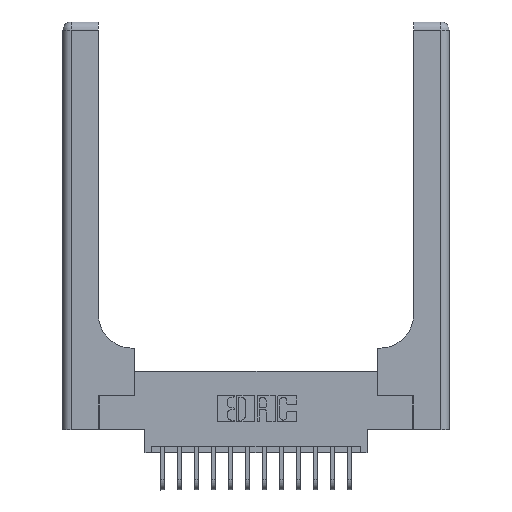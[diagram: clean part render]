
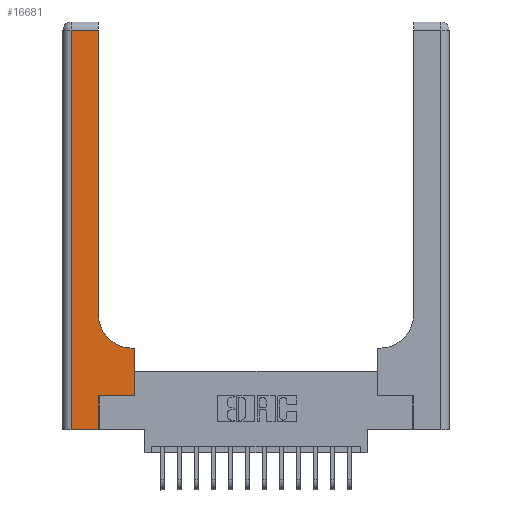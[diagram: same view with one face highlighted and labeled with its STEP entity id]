
A CAD part, top view. The second image highlights one B-rep face of the part: STEP entity #16681.
In plain terms, the highlighted planar face has unit normal (0, 0, 1).
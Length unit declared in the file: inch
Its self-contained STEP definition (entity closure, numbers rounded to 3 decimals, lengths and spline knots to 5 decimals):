
#87 = CARTESIAN_POINT ( 'NONE',  ( 0.528, 0.25, 0.37 ) ) ;
#623 = FACE_OUTER_BOUND ( 'NONE', #810, .T. ) ;
#810 = EDGE_LOOP ( 'NONE', ( #16310, #6818, #9333, #6764, #7889, #3598, #5517, #10188, #7358 ) ) ;
#1104 = LINE ( 'NONE', #11656, #10890 ) ;
#1242 = LINE ( 'NONE', #17725, #15218 ) ;
#1828 = EDGE_CURVE ( 'NONE', #3125, #15995, #2176, .T. ) ;
#2105 = PLANE ( 'NONE',  #14768 ) ;
#2176 = LINE ( 'NONE', #15721, #14375 ) ;
#2318 = DIRECTION ( 'NONE',  ( -1., 0., 0. ) ) ;
#2379 = CARTESIAN_POINT ( 'NONE',  ( 0.06, 2.94, 0.37 ) ) ;
#2805 = CARTESIAN_POINT ( 'NONE',  ( 0.265, 0., 0.37 ) ) ;
#3067 = CARTESIAN_POINT ( 'NONE',  ( 0.265, 0., 0.37 ) ) ;
#3098 = CARTESIAN_POINT ( 'NONE',  ( 0., 0., 0.37 ) ) ;
#3125 = VERTEX_POINT ( 'NONE', #10944 ) ;
#3320 = CARTESIAN_POINT ( 'NONE',  ( 0.26, 2.94, 0.37 ) ) ;
#3598 = ORIENTED_EDGE ( 'NONE', *, *, #18390, .T. ) ;
#4007 = CARTESIAN_POINT ( 'NONE',  ( 0.51, 0.6, 0.37 ) ) ;
#4327 = VERTEX_POINT ( 'NONE', #14497 ) ;
#5517 = ORIENTED_EDGE ( 'NONE', *, *, #10714, .T. ) ;
#5821 = VECTOR ( 'NONE', #13279, 39.37008 ) ;
#6764 = ORIENTED_EDGE ( 'NONE', *, *, #14956, .T. ) ;
#6818 = ORIENTED_EDGE ( 'NONE', *, *, #6959, .T. ) ;
#6959 = EDGE_CURVE ( 'NONE', #15995, #10327, #1104, .T. ) ;
#7268 = VECTOR ( 'NONE', #9680, 39.37008 ) ;
#7292 = DIRECTION ( 'NONE',  ( 0., 0., -1. ) ) ;
#7358 = ORIENTED_EDGE ( 'NONE', *, *, #9539, .T. ) ;
#7841 = VECTOR ( 'NONE', #12265, 39.37008 ) ;
#7850 = EDGE_CURVE ( 'NONE', #10327, #13882, #17471, .T. ) ;
#7889 = ORIENTED_EDGE ( 'NONE', *, *, #10748, .T. ) ;
#8124 = DIRECTION ( 'NONE',  ( 0., 0., -1. ) ) ;
#8308 = CARTESIAN_POINT ( 'NONE',  ( 0.265, 0.25, 0.37 ) ) ;
#8493 = VERTEX_POINT ( 'NONE', #4007 ) ;
#8628 = DIRECTION ( 'NONE',  ( 0., 1., 0. ) ) ;
#8700 = VECTOR ( 'NONE', #2318, 39.37008 ) ;
#9197 = DIRECTION ( 'NONE',  ( -1., 0., 0. ) ) ;
#9333 = ORIENTED_EDGE ( 'NONE', *, *, #7850, .T. ) ;
#9539 = EDGE_CURVE ( 'NONE', #8493, #3125, #19323, .T. ) ;
#9680 = DIRECTION ( 'NONE',  ( 1., 0., 0. ) ) ;
#10188 = ORIENTED_EDGE ( 'NONE', *, *, #11482, .T. ) ;
#10327 = VERTEX_POINT ( 'NONE', #2379 ) ;
#10426 = CARTESIAN_POINT ( 'NONE',  ( 0.06, 0., 0.37 ) ) ;
#10714 = EDGE_CURVE ( 'NONE', #18818, #4327, #1242, .T. ) ;
#10748 = EDGE_CURVE ( 'NONE', #12041, #18580, #17923, .T. ) ;
#10890 = VECTOR ( 'NONE', #16944, 39.37008 ) ;
#10944 = CARTESIAN_POINT ( 'NONE',  ( 0.26, 0.85, 0.37 ) ) ;
#11335 = DIRECTION ( 'NONE',  ( 0., 1., 0. ) ) ;
#11482 = EDGE_CURVE ( 'NONE', #4327, #8493, #15766, .T. ) ;
#11594 = CARTESIAN_POINT ( 'NONE',  ( 0.26, 0.6, 0.37 ) ) ;
#11625 = DIRECTION ( 'NONE',  ( 1., 0., 0. ) ) ;
#11656 = CARTESIAN_POINT ( 'NONE',  ( 0., 2.94, 0.37 ) ) ;
#11733 = CARTESIAN_POINT ( 'NONE',  ( 0.51, 0.85, 0.37 ) ) ;
#12041 = VERTEX_POINT ( 'NONE', #3067 ) ;
#12265 = DIRECTION ( 'NONE',  ( 1., 0., 0. ) ) ;
#12767 = AXIS2_PLACEMENT_3D ( 'NONE', #11733, #7292, #11625 ) ;
#13279 = DIRECTION ( 'NONE',  ( 0., 1., 0. ) ) ;
#13396 = CARTESIAN_POINT ( 'NONE',  ( 0.06, 3., 0.37 ) ) ;
#13712 = CARTESIAN_POINT ( 'NONE',  ( 0.265, 0.25, 0.37 ) ) ;
#13830 = CARTESIAN_POINT ( 'NONE',  ( 0., 3., 0.37 ) ) ;
#13882 = VERTEX_POINT ( 'NONE', #10426 ) ;
#14375 = VECTOR ( 'NONE', #11335, 39.37008 ) ;
#14497 = CARTESIAN_POINT ( 'NONE',  ( 0.528, 0.6, 0.37 ) ) ;
#14644 = DIRECTION ( 'NONE',  ( 0., -1., 0. ) ) ;
#14718 = VECTOR ( 'NONE', #14644, 39.37008 ) ;
#14768 = AXIS2_PLACEMENT_3D ( 'NONE', #13830, #8124, #9197 ) ;
#14956 = EDGE_CURVE ( 'NONE', #13882, #12041, #15449, .T. ) ;
#15218 = VECTOR ( 'NONE', #8628, 39.37008 ) ;
#15449 = LINE ( 'NONE', #3098, #7841 ) ;
#15721 = CARTESIAN_POINT ( 'NONE',  ( 0.26, 3., 0.37 ) ) ;
#15766 = LINE ( 'NONE', #11594, #8700 ) ;
#15995 = VERTEX_POINT ( 'NONE', #3320 ) ;
#16310 = ORIENTED_EDGE ( 'NONE', *, *, #1828, .T. ) ;
#16681 = ADVANCED_FACE ( 'NONE', ( #623 ), #2105, .F. ) ;
#16944 = DIRECTION ( 'NONE',  ( -1., 0., 0. ) ) ;
#17094 = LINE ( 'NONE', #8308, #7268 ) ;
#17471 = LINE ( 'NONE', #13396, #14718 ) ;
#17725 = CARTESIAN_POINT ( 'NONE',  ( 0.528, 0.25, 0.37 ) ) ;
#17923 = LINE ( 'NONE', #2805, #5821 ) ;
#18390 = EDGE_CURVE ( 'NONE', #18580, #18818, #17094, .T. ) ;
#18580 = VERTEX_POINT ( 'NONE', #13712 ) ;
#18818 = VERTEX_POINT ( 'NONE', #87 ) ;
#19323 = CIRCLE ( 'NONE', #12767, 0.25 ) ;
